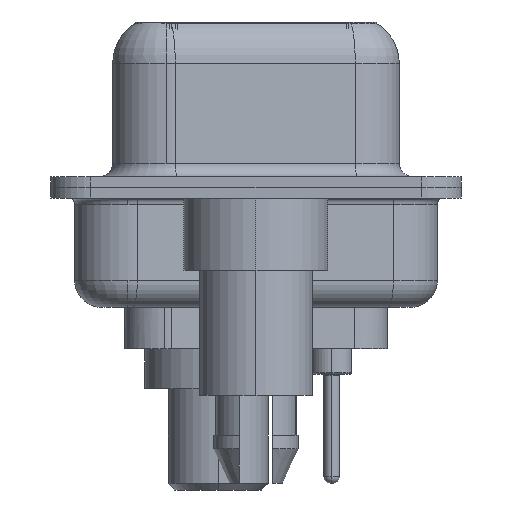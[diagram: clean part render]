
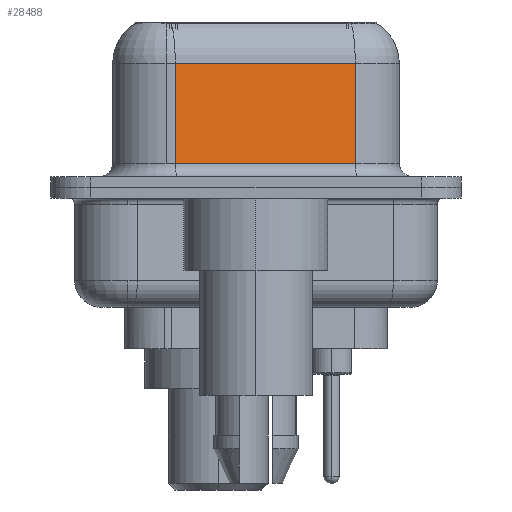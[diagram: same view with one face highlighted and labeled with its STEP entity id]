
A CAD part, left-side view. The second image highlights one B-rep face of the part: STEP entity #28488.
In plain terms, the highlighted planar face has unit normal (-0.985, -0.174, 0).
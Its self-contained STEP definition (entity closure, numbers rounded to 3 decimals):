
#758 = FACE_OUTER_BOUND ( 'NONE', #3578, .T. ) ;
#1470 = DIRECTION ( 'NONE',  ( 0.985, 0.174, 0. ) ) ;
#2403 = CARTESIAN_POINT ( 'NONE',  ( 5.621, -3.722, 4.65 ) ) ;
#2899 = DIRECTION ( 'NONE',  ( 0., 0., -1. ) ) ;
#3578 = EDGE_LOOP ( 'NONE', ( #12250, #32301, #30447, #7912 ) ) ;
#3949 = CARTESIAN_POINT ( 'NONE',  ( 4.43, 3.028, 4.65 ) ) ;
#4142 = CARTESIAN_POINT ( 'NONE',  ( 5.621, -3.722, 0.9 ) ) ;
#5426 = CARTESIAN_POINT ( 'NONE',  ( 5.621, -3.722, 4.65 ) ) ;
#6605 = EDGE_CURVE ( 'NONE', #9903, #25533, #33139, .T. ) ;
#6645 = VECTOR ( 'NONE', #33779, 1000. ) ;
#6968 = VERTEX_POINT ( 'NONE', #12577 ) ;
#7626 = VECTOR ( 'NONE', #2899, 1000. ) ;
#7912 = ORIENTED_EDGE ( 'NONE', *, *, #12690, .T. ) ;
#9903 = VERTEX_POINT ( 'NONE', #5426 ) ;
#10107 = AXIS2_PLACEMENT_3D ( 'NONE', #14882, #1470, #33175 ) ;
#10731 = LINE ( 'NONE', #2403, #6645 ) ;
#12250 = ORIENTED_EDGE ( 'NONE', *, *, #6605, .F. ) ;
#12466 = LINE ( 'NONE', #14135, #22709 ) ;
#12577 = CARTESIAN_POINT ( 'NONE',  ( 4.43, 3.028, 0.9 ) ) ;
#12690 = EDGE_CURVE ( 'NONE', #6968, #25533, #12466, .T. ) ;
#13437 = CARTESIAN_POINT ( 'NONE',  ( 4.43, 3.028, 6.4 ) ) ;
#13749 = VERTEX_POINT ( 'NONE', #3949 ) ;
#14135 = CARTESIAN_POINT ( 'NONE',  ( 5.621, -3.722, 0.9 ) ) ;
#14597 = EDGE_CURVE ( 'NONE', #9903, #13749, #10731, .T. ) ;
#14882 = CARTESIAN_POINT ( 'NONE',  ( 5.621, -3.722, 6.4 ) ) ;
#16364 = VECTOR ( 'NONE', #27011, 1000. ) ;
#18218 = EDGE_CURVE ( 'NONE', #13749, #6968, #33851, .T. ) ;
#19431 = DIRECTION ( 'NONE',  ( 0.174, -0.985, 0. ) ) ;
#22709 = VECTOR ( 'NONE', #19431, 1000. ) ;
#25533 = VERTEX_POINT ( 'NONE', #4142 ) ;
#26792 = CARTESIAN_POINT ( 'NONE',  ( 5.621, -3.722, 6.4 ) ) ;
#27011 = DIRECTION ( 'NONE',  ( 0., 0., -1. ) ) ;
#28488 = ADVANCED_FACE ( 'NONE', ( #758 ), #32840, .F. ) ;
#30447 = ORIENTED_EDGE ( 'NONE', *, *, #18218, .T. ) ;
#32301 = ORIENTED_EDGE ( 'NONE', *, *, #14597, .T. ) ;
#32840 = PLANE ( 'NONE',  #10107 ) ;
#33139 = LINE ( 'NONE', #26792, #16364 ) ;
#33175 = DIRECTION ( 'NONE',  ( -0.174, 0.985, 0. ) ) ;
#33779 = DIRECTION ( 'NONE',  ( -0.174, 0.985, 0. ) ) ;
#33851 = LINE ( 'NONE', #13437, #7626 ) ;
